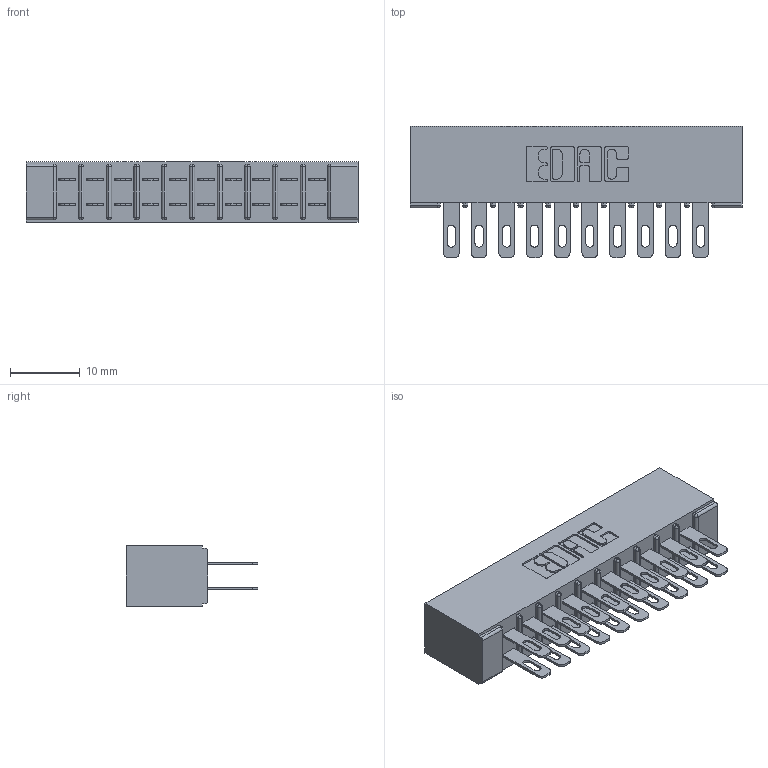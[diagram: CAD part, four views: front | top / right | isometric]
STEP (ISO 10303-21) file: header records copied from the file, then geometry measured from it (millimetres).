
FILE_DESCRIPTION (( 'STEP AP203' ), '1' );
FILE_NAME ('305-020-500-201.STEP', '2019-09-09T12:57:15', ( '' ), ( '' ), 'SwSTEP 2.0', 'SolidWorks 2016', '' );
FILE_SCHEMA (( 'CONFIG_CONTROL_DESIGN' ));
Length unit declared in the file: inch
Products named in the file (3): 305-290-001_500; 305 Part_No Mounting; 305-020-500-201
Assembly tree (21 placements, depth 2):
  305-020-500-201
    305 Part_No Mounting
    305-290-001_500  x20
Bounding box: 47.5 x 18.85 x 8.71 mm (x, y, z)
Volume: 3245.7 mm3; surface area: 6351.6 mm2
Topology: 21 solids, 21 shells, 1108 faces, 3162 edges, 2052 vertices
Faces by surface type: plane 624, cylinder 444, sphere 40
Entity records: 14467 total; most frequent: CARTESIAN_POINT 2392, ORIENTED_EDGE 2368, DIRECTION 2340, EDGE_CURVE 1184, LINE 924, VECTOR 924, VERTEX_POINT 760, AXIS2_PLACEMENT_3D 708
